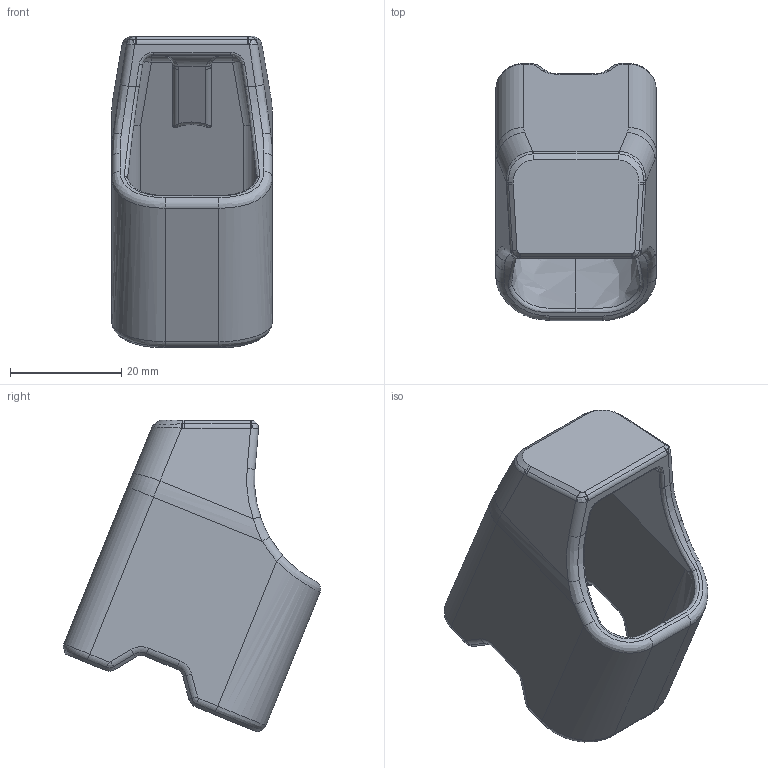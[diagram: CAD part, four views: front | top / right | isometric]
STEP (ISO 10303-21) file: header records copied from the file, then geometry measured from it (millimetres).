
FILE_DESCRIPTION(/* description */ (''),/* implementation_level */ '2;1');
FILE_NAME(/* name */ 'Glock Mag Loader.step',/* time_stamp */ '2021-03-16T15:37:41-04:00',/* author */ (''),/* organization */ (''),/* preprocessor_version */ 'ST-DEVELOPER v18.1',/* originating_system */ 'Autodesk Translation Framework v9.10.0.1330',/* authorisation */ '');
FILE_SCHEMA (('AUTOMOTIVE_DESIGN { 1 0 10303 214 3 1 1 }'));
Length unit declared in the file: millimetre
Products named in the file (1): Glock Mag Loader
Bounding box: 28.84 x 46.22 x 56.04 mm (x, y, z)
Volume: 13863.7 mm3; surface area: 10077 mm2
Topology: 1 solids, 1 shells, 279 faces, 656 edges, 370 vertices
Faces by surface type: bspline 88, cylinder 78, plane 65, cone 28, torus 20
Entity records: 10502 total; most frequent: CARTESIAN_POINT 4506, ORIENTED_EDGE 1296, DIRECTION 1164, EDGE_CURVE 648, AXIS2_PLACEMENT_3D 444, VERTEX_POINT 370, EDGE_LOOP 280, FACE_OUTER_BOUND 279
